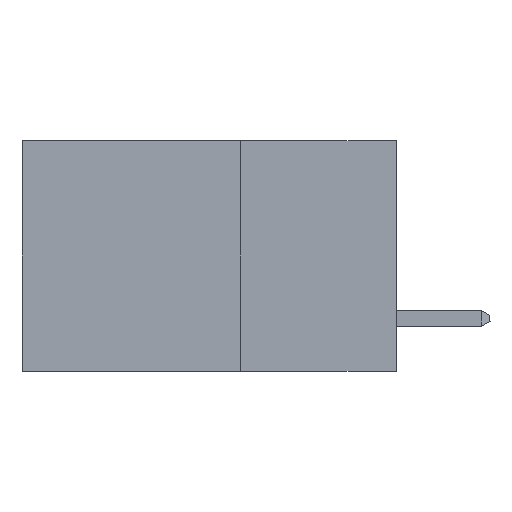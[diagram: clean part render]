
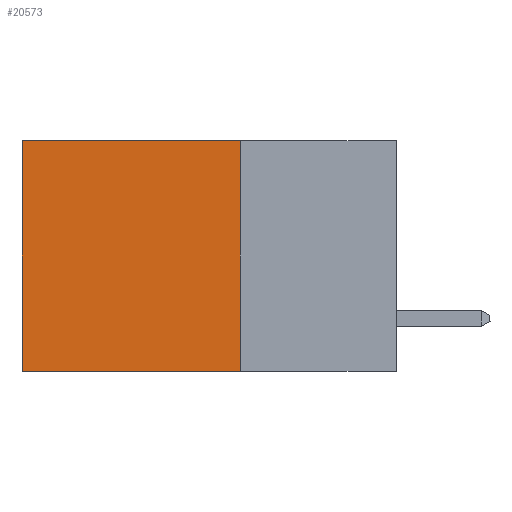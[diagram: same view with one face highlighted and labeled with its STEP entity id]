
A CAD part, left-side view. The second image highlights one B-rep face of the part: STEP entity #20573.
In plain terms, the highlighted planar face has unit normal (-1, 0, 0).
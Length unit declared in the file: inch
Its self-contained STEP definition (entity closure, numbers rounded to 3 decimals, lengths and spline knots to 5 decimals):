
#482 = CARTESIAN_POINT ( 'NONE',  ( 0.298, 0.6, -0.37 ) ) ;
#1117 = VERTEX_POINT ( 'NONE', #18100 ) ;
#1260 = VERTEX_POINT ( 'NONE', #12389 ) ;
#1601 = VECTOR ( 'NONE', #9292, 39.37008 ) ;
#3370 = CARTESIAN_POINT ( 'NONE',  ( 0.298, 0.25, -0.37 ) ) ;
#3414 = EDGE_CURVE ( 'NONE', #14759, #4048, #17668, .T. ) ;
#3611 = CARTESIAN_POINT ( 'NONE',  ( 0.298, 0.25, 0. ) ) ;
#4048 = VERTEX_POINT ( 'NONE', #482 ) ;
#6488 = ORIENTED_EDGE ( 'NONE', *, *, #21750, .T. ) ;
#7323 = LINE ( 'NONE', #3611, #16190 ) ;
#7593 = ORIENTED_EDGE ( 'NONE', *, *, #13397, .F. ) ;
#7703 = EDGE_LOOP ( 'NONE', ( #14737, #10149, #7593, #6488 ) ) ;
#8231 = CARTESIAN_POINT ( 'NONE',  ( 0.298, 0.25, 0. ) ) ;
#9137 = DIRECTION ( 'NONE',  ( 0., 1., 0. ) ) ;
#9292 = DIRECTION ( 'NONE',  ( 0., 0., -1. ) ) ;
#10149 = ORIENTED_EDGE ( 'NONE', *, *, #24242, .F. ) ;
#10160 = DIRECTION ( 'NONE',  ( 0., 0., -1. ) ) ;
#11830 = LINE ( 'NONE', #16803, #1601 ) ;
#12389 = CARTESIAN_POINT ( 'NONE',  ( 0.298, 0.25, 0. ) ) ;
#12685 = VECTOR ( 'NONE', #23781, 39.37008 ) ;
#12817 = VECTOR ( 'NONE', #9137, 39.37008 ) ;
#13397 = EDGE_CURVE ( 'NONE', #1260, #1117, #11830, .T. ) ;
#13904 = FACE_OUTER_BOUND ( 'NONE', #7703, .T. ) ;
#14737 = ORIENTED_EDGE ( 'NONE', *, *, #3414, .T. ) ;
#14759 = VERTEX_POINT ( 'NONE', #15185 ) ;
#15185 = CARTESIAN_POINT ( 'NONE',  ( 0.298, 0.6, 0. ) ) ;
#15787 = PLANE ( 'NONE',  #19969 ) ;
#16190 = VECTOR ( 'NONE', #24268, 39.37008 ) ;
#16803 = CARTESIAN_POINT ( 'NONE',  ( 0.298, 0.25, 0. ) ) ;
#17668 = LINE ( 'NONE', #22039, #12685 ) ;
#18100 = CARTESIAN_POINT ( 'NONE',  ( 0.298, 0.25, -0.37 ) ) ;
#19969 = AXIS2_PLACEMENT_3D ( 'NONE', #8231, #21334, #10160 ) ;
#20573 = ADVANCED_FACE ( 'NONE', ( #13904 ), #15787, .F. ) ;
#21334 = DIRECTION ( 'NONE',  ( 1., 0., 0. ) ) ;
#21750 = EDGE_CURVE ( 'NONE', #1260, #14759, #7323, .T. ) ;
#22039 = CARTESIAN_POINT ( 'NONE',  ( 0.298, 0.6, 0. ) ) ;
#23277 = LINE ( 'NONE', #3370, #12817 ) ;
#23781 = DIRECTION ( 'NONE',  ( 0., 0., -1. ) ) ;
#24242 = EDGE_CURVE ( 'NONE', #1117, #4048, #23277, .T. ) ;
#24268 = DIRECTION ( 'NONE',  ( 0., 1., 0. ) ) ;
